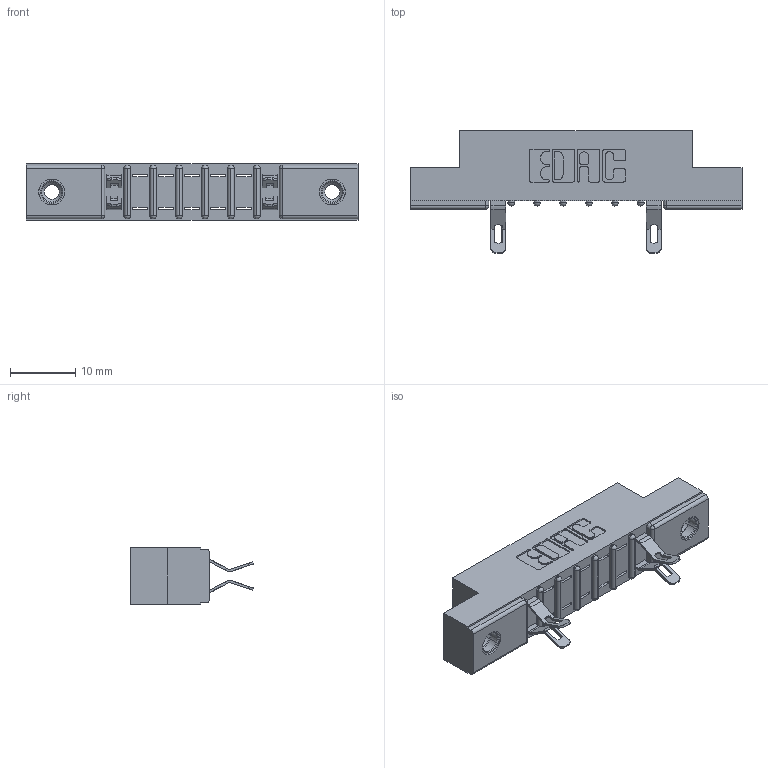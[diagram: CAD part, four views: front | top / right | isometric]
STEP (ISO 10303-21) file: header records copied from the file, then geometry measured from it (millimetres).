
FILE_DESCRIPTION (( 'STEP AP203' ), '1' );
FILE_NAME ('357-014-555-208.STEP', '2018-08-08T00:28:02', ( '' ), ( '' ), 'SwSTEP 2.0', 'SolidWorks 2016', '' );
FILE_SCHEMA (( 'CONFIG_CONTROL_DESIGN' ));
Length unit declared in the file: inch
Products named in the file (4): 345-250-001_345-250-003-102; 357-014-555-208; 307 Part_.156 Dia Mounting Holes; 307-290-001_555
Assembly tree (7 placements, depth 2):
  357-014-555-208
    307 Part_.156 Dia Mounting Holes
    307-290-001_555  x4
    345-250-001_345-250-003-102  x2
Bounding box: 50.75 x 18.75 x 8.71 mm (x, y, z)
Volume: 3197.1 mm3; surface area: 4187.6 mm2
Topology: 7 solids, 7 shells, 530 faces, 1503 edges, 966 vertices
Faces by surface type: plane 298, cylinder 200, sphere 16, cone 12, torus 4
Entity records: 11942 total; most frequent: CARTESIAN_POINT 1996, ORIENTED_EDGE 1980, DIRECTION 1976, EDGE_CURVE 990, VECTOR 732, LINE 732, VERTEX_POINT 642, AXIS2_PLACEMENT_3D 622
